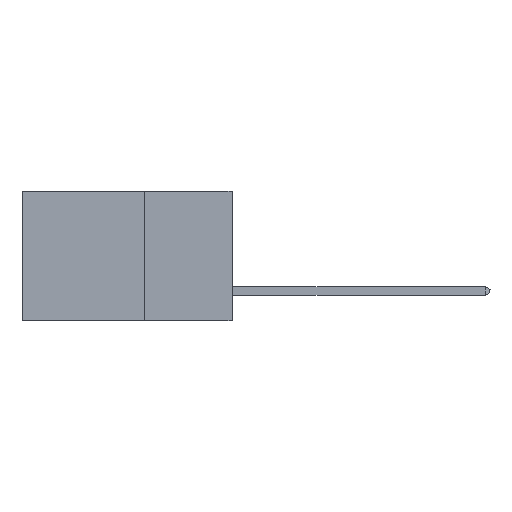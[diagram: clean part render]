
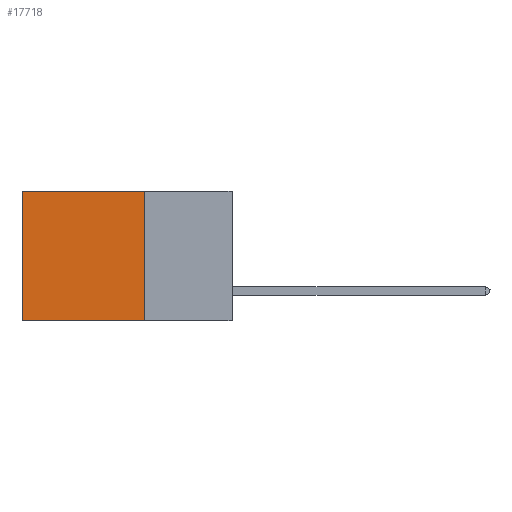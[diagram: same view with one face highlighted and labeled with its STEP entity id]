
A CAD part, left-side view. The second image highlights one B-rep face of the part: STEP entity #17718.
In plain terms, the highlighted planar face has unit normal (-1, 0, 0).
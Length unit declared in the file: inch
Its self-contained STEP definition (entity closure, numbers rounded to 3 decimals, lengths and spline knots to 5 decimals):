
#2246 = EDGE_CURVE ( 'NONE', #37318, #14053, #20031, .T. ) ;
#2606 = VECTOR ( 'NONE', #15459, 39.37008 ) ;
#6144 = ORIENTED_EDGE ( 'NONE', *, *, #19979, .F. ) ;
#8065 = CARTESIAN_POINT ( 'NONE',  ( 0.2875, 0.25, 0. ) ) ;
#8694 = VECTOR ( 'NONE', #27153, 39.37008 ) ;
#8941 = VERTEX_POINT ( 'NONE', #38848 ) ;
#11699 = CARTESIAN_POINT ( 'NONE',  ( 0.2875, 0.6, -0.37 ) ) ;
#14053 = VERTEX_POINT ( 'NONE', #39650 ) ;
#15459 = DIRECTION ( 'NONE',  ( 0., 1., 0. ) ) ;
#15576 = DIRECTION ( 'NONE',  ( 0., 1., 0. ) ) ;
#16499 = LINE ( 'NONE', #20277, #8694 ) ;
#17718 = ADVANCED_FACE ( 'NONE', ( #32070 ), #18014, .F. ) ;
#18014 = PLANE ( 'NONE',  #39481 ) ;
#18153 = DIRECTION ( 'NONE',  ( 1., 0., 0. ) ) ;
#18669 = CARTESIAN_POINT ( 'NONE',  ( 0.2875, 0.25, 0. ) ) ;
#18766 = ORIENTED_EDGE ( 'NONE', *, *, #42191, .T. ) ;
#19050 = ORIENTED_EDGE ( 'NONE', *, *, #30772, .T. ) ;
#19612 = VERTEX_POINT ( 'NONE', #11699 ) ;
#19979 = EDGE_CURVE ( 'NONE', #14053, #19612, #33505, .T. ) ;
#20031 = LINE ( 'NONE', #41800, #34735 ) ;
#20277 = CARTESIAN_POINT ( 'NONE',  ( 0.2875, 0.6, 0. ) ) ;
#22323 = CARTESIAN_POINT ( 'NONE',  ( 0.2875, 0.25, -0.37 ) ) ;
#23036 = VECTOR ( 'NONE', #15576, 39.37008 ) ;
#26737 = EDGE_LOOP ( 'NONE', ( #19050, #6144, #42776, #18766 ) ) ;
#27153 = DIRECTION ( 'NONE',  ( 0., 0., -1. ) ) ;
#28222 = LINE ( 'NONE', #18669, #2606 ) ;
#30772 = EDGE_CURVE ( 'NONE', #8941, #19612, #16499, .T. ) ;
#32070 = FACE_OUTER_BOUND ( 'NONE', #26737, .T. ) ;
#33505 = LINE ( 'NONE', #22323, #23036 ) ;
#34735 = VECTOR ( 'NONE', #42104, 39.37008 ) ;
#35373 = CARTESIAN_POINT ( 'NONE',  ( 0.2875, 0.25, 0. ) ) ;
#37318 = VERTEX_POINT ( 'NONE', #35373 ) ;
#38848 = CARTESIAN_POINT ( 'NONE',  ( 0.2875, 0.6, 0. ) ) ;
#39481 = AXIS2_PLACEMENT_3D ( 'NONE', #8065, #18153, #41623 ) ;
#39650 = CARTESIAN_POINT ( 'NONE',  ( 0.2875, 0.25, -0.37 ) ) ;
#41623 = DIRECTION ( 'NONE',  ( 0., 0., -1. ) ) ;
#41800 = CARTESIAN_POINT ( 'NONE',  ( 0.2875, 0.25, 0. ) ) ;
#42104 = DIRECTION ( 'NONE',  ( 0., 0., -1. ) ) ;
#42191 = EDGE_CURVE ( 'NONE', #37318, #8941, #28222, .T. ) ;
#42776 = ORIENTED_EDGE ( 'NONE', *, *, #2246, .F. ) ;
